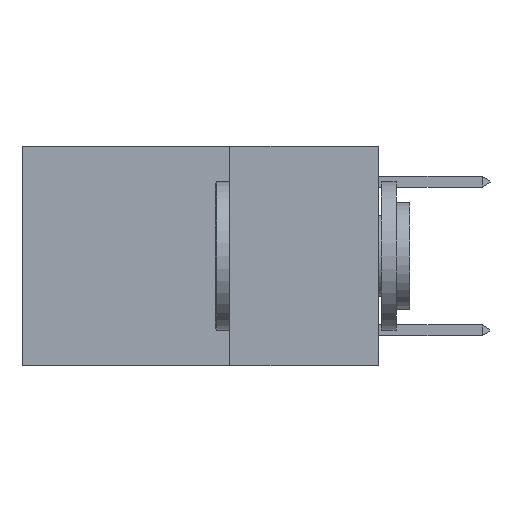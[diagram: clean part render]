
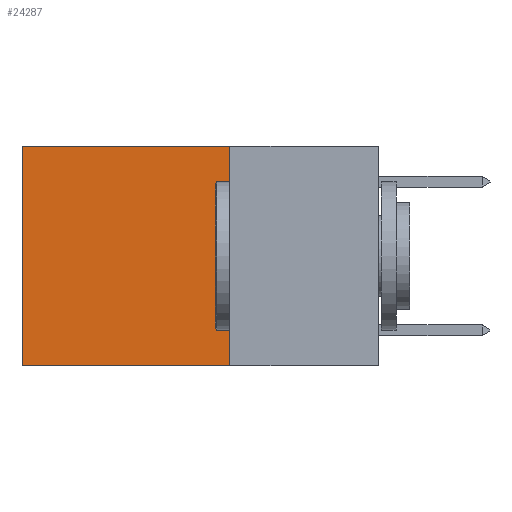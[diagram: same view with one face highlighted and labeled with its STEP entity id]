
A CAD part, left-side view. The second image highlights one B-rep face of the part: STEP entity #24287.
In plain terms, the highlighted planar face has unit normal (-1, 0, 0).
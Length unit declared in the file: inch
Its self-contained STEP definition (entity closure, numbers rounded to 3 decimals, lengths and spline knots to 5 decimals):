
#591 = CARTESIAN_POINT ( 'NONE',  ( 0.2625, 0.25, 0. ) ) ;
#896 = VECTOR ( 'NONE', #2299, 39.37008 ) ;
#1619 = CARTESIAN_POINT ( 'NONE',  ( 0.2625, 0.25, 0. ) ) ;
#1888 = DIRECTION ( 'NONE',  ( 0., 1., 0. ) ) ;
#2299 = DIRECTION ( 'NONE',  ( 0., 0., -1. ) ) ;
#3224 = VECTOR ( 'NONE', #3965, 39.37008 ) ;
#3429 = EDGE_LOOP ( 'NONE', ( #27170, #4413, #26884, #24368 ) ) ;
#3965 = DIRECTION ( 'NONE',  ( 0., 1., 0. ) ) ;
#4413 = ORIENTED_EDGE ( 'NONE', *, *, #15383, .F. ) ;
#7026 = CARTESIAN_POINT ( 'NONE',  ( 0.2625, 0.25, -0.37 ) ) ;
#7136 = VERTEX_POINT ( 'NONE', #27825 ) ;
#7667 = EDGE_CURVE ( 'NONE', #27009, #7136, #20517, .T. ) ;
#8599 = FACE_OUTER_BOUND ( 'NONE', #3429, .T. ) ;
#9634 = CARTESIAN_POINT ( 'NONE',  ( 0.2625, 0.25, -0.37 ) ) ;
#10414 = EDGE_CURVE ( 'NONE', #7136, #26726, #30469, .T. ) ;
#11634 = VECTOR ( 'NONE', #30034, 39.37008 ) ;
#15340 = CARTESIAN_POINT ( 'NONE',  ( 0.2625, 0.25, 0. ) ) ;
#15383 = EDGE_CURVE ( 'NONE', #17273, #26726, #23235, .T. ) ;
#16038 = EDGE_CURVE ( 'NONE', #27009, #17273, #20593, .T. ) ;
#16095 = PLANE ( 'NONE',  #16412 ) ;
#16183 = CARTESIAN_POINT ( 'NONE',  ( 0.2625, 0.6, 0. ) ) ;
#16412 = AXIS2_PLACEMENT_3D ( 'NONE', #1619, #17968, #22785 ) ;
#17273 = VERTEX_POINT ( 'NONE', #9634 ) ;
#17923 = CARTESIAN_POINT ( 'NONE',  ( 0.2625, 0.25, 0. ) ) ;
#17968 = DIRECTION ( 'NONE',  ( 1., 0., 0. ) ) ;
#18816 = CARTESIAN_POINT ( 'NONE',  ( 0.2625, 0.6, -0.37 ) ) ;
#20517 = LINE ( 'NONE', #15340, #3224 ) ;
#20593 = LINE ( 'NONE', #17923, #11634 ) ;
#22785 = DIRECTION ( 'NONE',  ( 0., 0., -1. ) ) ;
#23235 = LINE ( 'NONE', #7026, #24154 ) ;
#24154 = VECTOR ( 'NONE', #1888, 39.37008 ) ;
#24287 = ADVANCED_FACE ( 'NONE', ( #8599 ), #16095, .F. ) ;
#24368 = ORIENTED_EDGE ( 'NONE', *, *, #7667, .T. ) ;
#26726 = VERTEX_POINT ( 'NONE', #18816 ) ;
#26884 = ORIENTED_EDGE ( 'NONE', *, *, #16038, .F. ) ;
#27009 = VERTEX_POINT ( 'NONE', #591 ) ;
#27170 = ORIENTED_EDGE ( 'NONE', *, *, #10414, .T. ) ;
#27825 = CARTESIAN_POINT ( 'NONE',  ( 0.2625, 0.6, 0. ) ) ;
#30034 = DIRECTION ( 'NONE',  ( 0., 0., -1. ) ) ;
#30469 = LINE ( 'NONE', #16183, #896 ) ;
